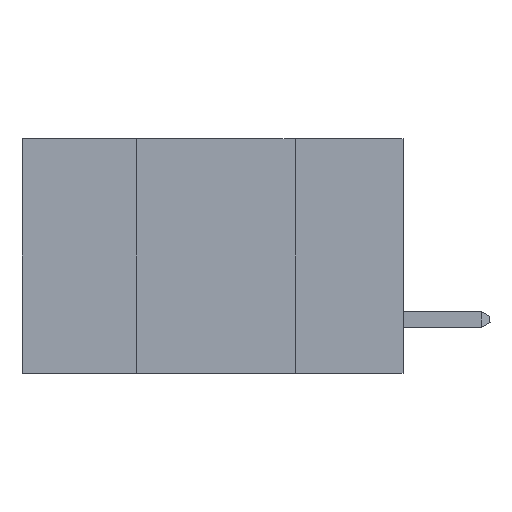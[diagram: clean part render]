
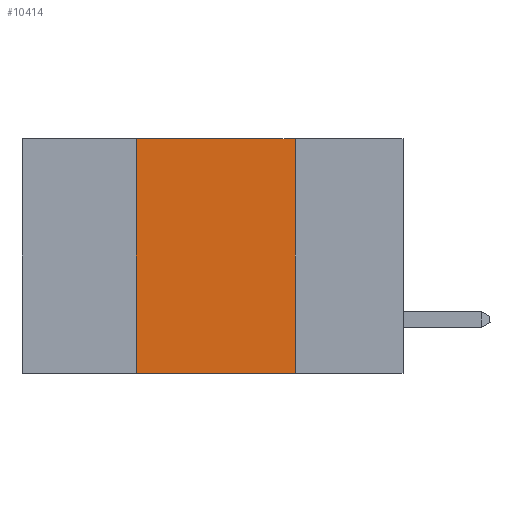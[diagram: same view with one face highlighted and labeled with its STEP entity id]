
A CAD part, left-side view. The second image highlights one B-rep face of the part: STEP entity #10414.
In plain terms, the highlighted planar face has unit normal (-1, 0, 0).
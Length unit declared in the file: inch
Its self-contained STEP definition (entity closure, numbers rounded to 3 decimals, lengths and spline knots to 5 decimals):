
#397 = EDGE_CURVE ( 'NONE', #7111, #22292, #9715, .T. ) ;
#1316 = CARTESIAN_POINT ( 'NONE',  ( 0., 0.17, 0. ) ) ;
#1539 = ORIENTED_EDGE ( 'NONE', *, *, #14747, .F. ) ;
#2542 = VECTOR ( 'NONE', #10643, 39.37008 ) ;
#4279 = DIRECTION ( 'NONE',  ( 0., 0., 1. ) ) ;
#5468 = VECTOR ( 'NONE', #19387, 39.37008 ) ;
#5803 = VERTEX_POINT ( 'NONE', #21342 ) ;
#6151 = VERTEX_POINT ( 'NONE', #20512 ) ;
#6687 = CARTESIAN_POINT ( 'NONE',  ( 0., 0.17, 0. ) ) ;
#7111 = VERTEX_POINT ( 'NONE', #15266 ) ;
#8065 = FACE_OUTER_BOUND ( 'NONE', #24732, .T. ) ;
#8893 = ORIENTED_EDGE ( 'NONE', *, *, #19824, .T. ) ;
#9568 = DIRECTION ( 'NONE',  ( 0., 0., -1. ) ) ;
#9715 = LINE ( 'NONE', #13161, #5468 ) ;
#10095 = CARTESIAN_POINT ( 'NONE',  ( 0., 0.42, 0. ) ) ;
#10414 = ADVANCED_FACE ( 'NONE', ( #8065 ), #23154, .F. ) ;
#10643 = DIRECTION ( 'NONE',  ( 0., 0., -1. ) ) ;
#10925 = EDGE_CURVE ( 'NONE', #22292, #5803, #21352, .T. ) ;
#11489 = DIRECTION ( 'NONE',  ( 1., 0., 0. ) ) ;
#12612 = ORIENTED_EDGE ( 'NONE', *, *, #397, .F. ) ;
#13161 = CARTESIAN_POINT ( 'NONE',  ( 0., 0.6, 0. ) ) ;
#14747 = EDGE_CURVE ( 'NONE', #6151, #7111, #23631, .T. ) ;
#15255 = CARTESIAN_POINT ( 'NONE',  ( 0., 0.6, 0. ) ) ;
#15266 = CARTESIAN_POINT ( 'NONE',  ( 0., 0.42, 0. ) ) ;
#17054 = AXIS2_PLACEMENT_3D ( 'NONE', #15255, #11489, #9568 ) ;
#18834 = LINE ( 'NONE', #21517, #20710 ) ;
#19387 = DIRECTION ( 'NONE',  ( 0., -1., 0. ) ) ;
#19824 = EDGE_CURVE ( 'NONE', #6151, #5803, #18834, .T. ) ;
#20512 = CARTESIAN_POINT ( 'NONE',  ( 0., 0.42, -0.37 ) ) ;
#20710 = VECTOR ( 'NONE', #23592, 39.37008 ) ;
#21342 = CARTESIAN_POINT ( 'NONE',  ( 0., 0.17, -0.37 ) ) ;
#21352 = LINE ( 'NONE', #6687, #2542 ) ;
#21517 = CARTESIAN_POINT ( 'NONE',  ( 0., 0.6, -0.37 ) ) ;
#22292 = VERTEX_POINT ( 'NONE', #1316 ) ;
#23154 = PLANE ( 'NONE',  #17054 ) ;
#23340 = VECTOR ( 'NONE', #4279, 39.37008 ) ;
#23592 = DIRECTION ( 'NONE',  ( 0., -1., 0. ) ) ;
#23631 = LINE ( 'NONE', #10095, #23340 ) ;
#24652 = ORIENTED_EDGE ( 'NONE', *, *, #10925, .F. ) ;
#24732 = EDGE_LOOP ( 'NONE', ( #24652, #12612, #1539, #8893 ) ) ;
